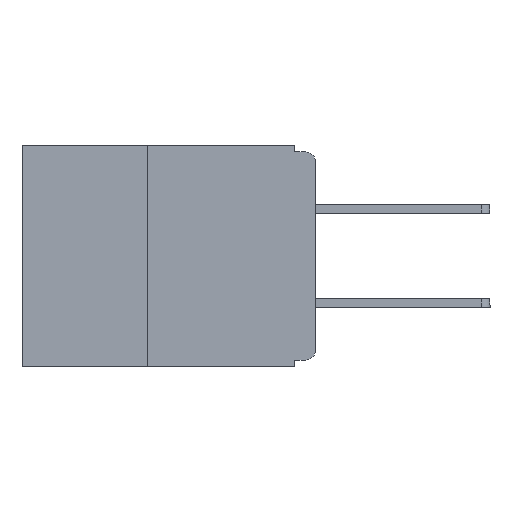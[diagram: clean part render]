
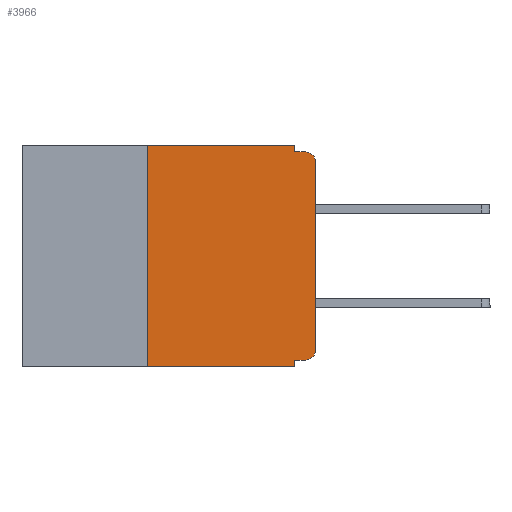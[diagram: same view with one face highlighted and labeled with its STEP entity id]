
A CAD part, left-side view. The second image highlights one B-rep face of the part: STEP entity #3966.
In plain terms, the highlighted planar face has unit normal (-1, 0, 0).
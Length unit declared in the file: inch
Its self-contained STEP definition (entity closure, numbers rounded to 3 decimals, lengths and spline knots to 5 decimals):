
#17 = DIRECTION ( 'NONE',  ( 0., 0., -1. ) ) ;
#51 = DIRECTION ( 'NONE',  ( 0., -1., 0. ) ) ;
#635 = VERTEX_POINT ( 'NONE', #25798 ) ;
#872 = DIRECTION ( 'NONE',  ( 0., -1., 0. ) ) ;
#1189 = EDGE_CURVE ( 'NONE', #10382, #22716, #29756, .T. ) ;
#1204 = ORIENTED_EDGE ( 'NONE', *, *, #14831, .F. ) ;
#1271 = VERTEX_POINT ( 'NONE', #1698 ) ;
#1414 = ORIENTED_EDGE ( 'NONE', *, *, #4599, .T. ) ;
#1486 = ORIENTED_EDGE ( 'NONE', *, *, #10991, .F. ) ;
#1678 = EDGE_CURVE ( 'NONE', #635, #26978, #17141, .T. ) ;
#1698 = CARTESIAN_POINT ( 'NONE',  ( 0., 0., -0.305 ) ) ;
#2004 = CIRCLE ( 'NONE', #7862, 0.015 ) ;
#2312 = ORIENTED_EDGE ( 'NONE', *, *, #1189, .T. ) ;
#2733 = EDGE_CURVE ( 'NONE', #13835, #19101, #12680, .T. ) ;
#2967 = LINE ( 'NONE', #27397, #27333 ) ;
#3388 = EDGE_CURVE ( 'NONE', #13927, #21219, #20737, .T. ) ;
#3966 = ADVANCED_FACE ( 'NONE', ( #21060 ), #14428, .F. ) ;
#4599 = EDGE_CURVE ( 'NONE', #1271, #13835, #2967, .T. ) ;
#5250 = ORIENTED_EDGE ( 'NONE', *, *, #2733, .T. ) ;
#5643 = CARTESIAN_POINT ( 'NONE',  ( 0., 0.015, -0.01 ) ) ;
#6872 = CARTESIAN_POINT ( 'NONE',  ( 0., 0.031, -0.01 ) ) ;
#6901 = DIRECTION ( 'NONE',  ( 0., 0., 1. ) ) ;
#7862 = AXIS2_PLACEMENT_3D ( 'NONE', #9000, #25400, #11337 ) ;
#9000 = CARTESIAN_POINT ( 'NONE',  ( 0., 0.015, -0.305 ) ) ;
#10339 = DIRECTION ( 'NONE',  ( 0., 0., -1. ) ) ;
#10382 = VERTEX_POINT ( 'NONE', #16674 ) ;
#10730 = LINE ( 'NONE', #11877, #23978 ) ;
#10906 = VECTOR ( 'NONE', #22768, 39.37008 ) ;
#10991 = EDGE_CURVE ( 'NONE', #26978, #22716, #27657, .T. ) ;
#11104 = VECTOR ( 'NONE', #872, 39.37008 ) ;
#11337 = DIRECTION ( 'NONE',  ( 0., 0., -1. ) ) ;
#11359 = CARTESIAN_POINT ( 'NONE',  ( 0., 0.031, 0. ) ) ;
#11440 = DIRECTION ( 'NONE',  ( 0., 0., -1. ) ) ;
#11463 = DIRECTION ( 'NONE',  ( -1., 0., 0. ) ) ;
#11471 = CARTESIAN_POINT ( 'NONE',  ( 0., 0.015, -0.025 ) ) ;
#11877 = CARTESIAN_POINT ( 'NONE',  ( 0., 0.437, 0. ) ) ;
#11948 = CARTESIAN_POINT ( 'NONE',  ( 0., 0., -0.01 ) ) ;
#12680 = CIRCLE ( 'NONE', #19027, 0.015 ) ;
#13775 = DIRECTION ( 'NONE',  ( 0., 0., -1. ) ) ;
#13835 = VERTEX_POINT ( 'NONE', #19625 ) ;
#13836 = DIRECTION ( 'NONE',  ( 1., 0., 0. ) ) ;
#13927 = VERTEX_POINT ( 'NONE', #29313 ) ;
#14216 = CARTESIAN_POINT ( 'NONE',  ( 0., 0.437, 0. ) ) ;
#14428 = PLANE ( 'NONE',  #18271 ) ;
#14706 = VECTOR ( 'NONE', #51, 39.37008 ) ;
#14816 = CARTESIAN_POINT ( 'NONE',  ( 0., 0.031, -0.32 ) ) ;
#14831 = EDGE_CURVE ( 'NONE', #17611, #13927, #10730, .T. ) ;
#16603 = VECTOR ( 'NONE', #17, 39.37008 ) ;
#16637 = CARTESIAN_POINT ( 'NONE',  ( 0., 0.031, -0.33 ) ) ;
#16674 = CARTESIAN_POINT ( 'NONE',  ( 0., 0.25, -0.33 ) ) ;
#17141 = LINE ( 'NONE', #24472, #10906 ) ;
#17611 = VERTEX_POINT ( 'NONE', #18183 ) ;
#17849 = ORIENTED_EDGE ( 'NONE', *, *, #1678, .F. ) ;
#18183 = CARTESIAN_POINT ( 'NONE',  ( 0., 0.25, 0. ) ) ;
#18271 = AXIS2_PLACEMENT_3D ( 'NONE', #14216, #13836, #13775 ) ;
#19027 = AXIS2_PLACEMENT_3D ( 'NONE', #11471, #11463, #11440 ) ;
#19101 = VERTEX_POINT ( 'NONE', #5643 ) ;
#19625 = CARTESIAN_POINT ( 'NONE',  ( 0., 0., -0.025 ) ) ;
#20737 = LINE ( 'NONE', #11359, #25493 ) ;
#20899 = VECTOR ( 'NONE', #6901, 39.37008 ) ;
#21060 = FACE_OUTER_BOUND ( 'NONE', #29224, .T. ) ;
#21219 = VERTEX_POINT ( 'NONE', #6872 ) ;
#21349 = ORIENTED_EDGE ( 'NONE', *, *, #29367, .F. ) ;
#22023 = DIRECTION ( 'NONE',  ( 0., 0., 1. ) ) ;
#22359 = ORIENTED_EDGE ( 'NONE', *, *, #23744, .T. ) ;
#22716 = VERTEX_POINT ( 'NONE', #28588 ) ;
#22768 = DIRECTION ( 'NONE',  ( 0., 1., 0. ) ) ;
#23164 = ORIENTED_EDGE ( 'NONE', *, *, #3388, .F. ) ;
#23311 = CARTESIAN_POINT ( 'NONE',  ( 0., 0.25, -0.33 ) ) ;
#23553 = CARTESIAN_POINT ( 'NONE',  ( 0., 0.437, -0.33 ) ) ;
#23744 = EDGE_CURVE ( 'NONE', #635, #1271, #2004, .T. ) ;
#23978 = VECTOR ( 'NONE', #28313, 39.37008 ) ;
#24472 = CARTESIAN_POINT ( 'NONE',  ( 0., 0., -0.32 ) ) ;
#25400 = DIRECTION ( 'NONE',  ( -1., 0., 0. ) ) ;
#25493 = VECTOR ( 'NONE', #10339, 39.37008 ) ;
#25798 = CARTESIAN_POINT ( 'NONE',  ( 0., 0.015, -0.32 ) ) ;
#25984 = ORIENTED_EDGE ( 'NONE', *, *, #28565, .F. ) ;
#26978 = VERTEX_POINT ( 'NONE', #14816 ) ;
#27172 = LINE ( 'NONE', #23311, #20899 ) ;
#27229 = LINE ( 'NONE', #11948, #14706 ) ;
#27333 = VECTOR ( 'NONE', #22023, 39.37008 ) ;
#27397 = CARTESIAN_POINT ( 'NONE',  ( 0., 0., 0. ) ) ;
#27657 = LINE ( 'NONE', #16637, #16603 ) ;
#28313 = DIRECTION ( 'NONE',  ( 0., -1., 0. ) ) ;
#28565 = EDGE_CURVE ( 'NONE', #21219, #19101, #27229, .T. ) ;
#28588 = CARTESIAN_POINT ( 'NONE',  ( 0., 0.031, -0.33 ) ) ;
#29224 = EDGE_LOOP ( 'NONE', ( #1414, #5250, #25984, #23164, #1204, #21349, #2312, #1486, #17849, #22359 ) ) ;
#29313 = CARTESIAN_POINT ( 'NONE',  ( 0., 0.031, 0. ) ) ;
#29367 = EDGE_CURVE ( 'NONE', #10382, #17611, #27172, .T. ) ;
#29756 = LINE ( 'NONE', #23553, #11104 ) ;
